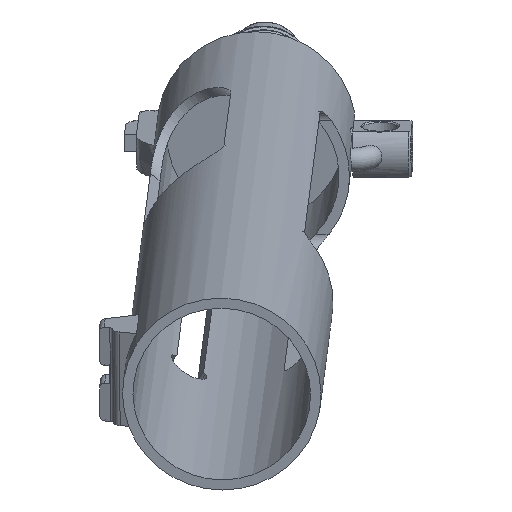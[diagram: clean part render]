
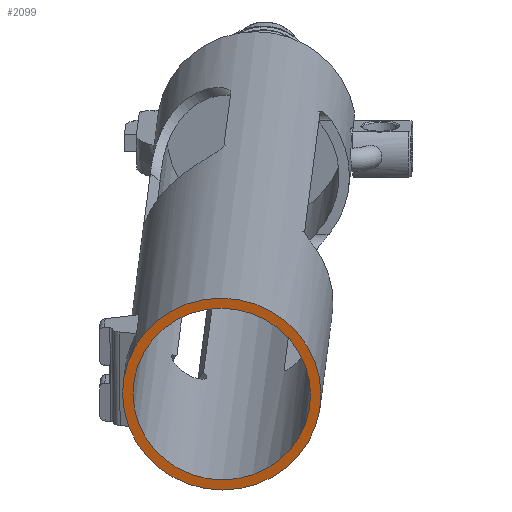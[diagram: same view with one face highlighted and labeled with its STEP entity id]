
A CAD part, left-side view. The second image highlights one B-rep face of the part: STEP entity #2099.
In plain terms, the highlighted planar face has unit normal (-0.965, 0.034, -0.259).
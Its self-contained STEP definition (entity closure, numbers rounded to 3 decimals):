
#83=PLANE('',#2297);
#111=FACE_BOUND('',#645,.T.);
#515=FACE_OUTER_BOUND('',#644,.T.);
#644=EDGE_LOOP('',(#1923));
#645=EDGE_LOOP('',(#1924));
#814=CIRCLE('',#2239,19.05);
#818=CIRCLE('',#2247,17.05);
#962=VERTEX_POINT('',#13615);
#984=VERTEX_POINT('',#13812);
#1233=EDGE_CURVE('',#962,#962,#814,.T.);
#1258=EDGE_CURVE('',#984,#984,#818,.T.);
#1923=ORIENTED_EDGE('',*,*,#1233,.F.);
#1924=ORIENTED_EDGE('',*,*,#1258,.F.);
#2099=ADVANCED_FACE('',(#515,#111),#83,.F.);
#2239=AXIS2_PLACEMENT_3D('',#13617,#2583,#2584);
#2247=AXIS2_PLACEMENT_3D('',#13814,#2609,#2610);
#2297=AXIS2_PLACEMENT_3D('',#14139,#2752,#2753);
#2583=DIRECTION('center_axis',(0.965,-0.034,0.259));
#2584=DIRECTION('ref_axis',(0.261,0.165,-0.951));
#2609=DIRECTION('center_axis',(-0.965,0.034,-0.259));
#2610=DIRECTION('ref_axis',(-0.261,-0.165,0.951));
#2752=DIRECTION('center_axis',(0.965,-0.034,0.259));
#2753=DIRECTION('ref_axis',(0.011,-0.986,-0.168));
#13615=CARTESIAN_POINT('',(-687.528,357.31,-2349.026));
#13617=CARTESIAN_POINT('Origin',(-682.56,360.446,-2367.148));
#13812=CARTESIAN_POINT('',(-678.113,363.253,-2383.366));
#13814=CARTESIAN_POINT('Origin',(-682.56,360.446,-2367.148));
#14139=CARTESIAN_POINT('Origin',(-682.56,360.446,-2367.148));
